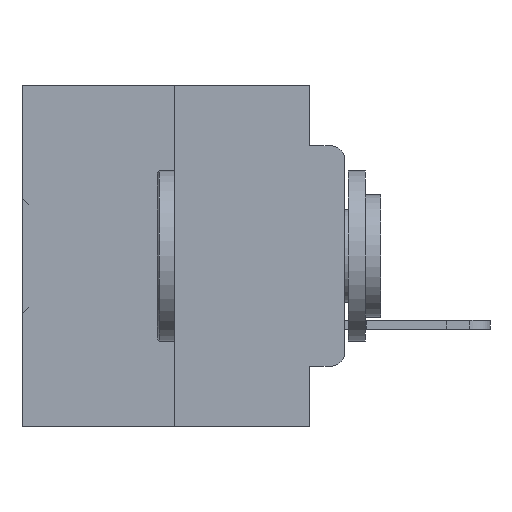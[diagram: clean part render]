
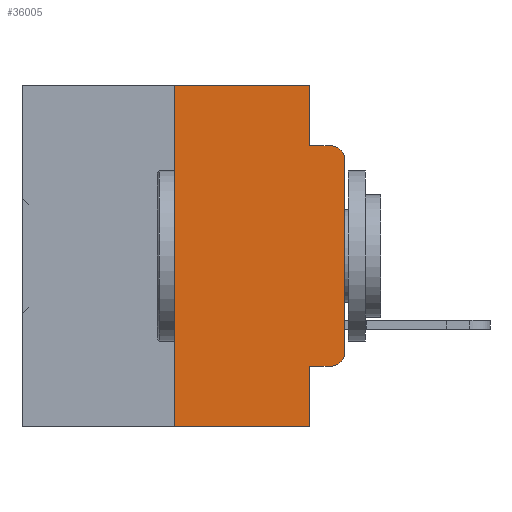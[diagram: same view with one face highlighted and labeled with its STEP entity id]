
A CAD part, left-side view. The second image highlights one B-rep face of the part: STEP entity #36005.
In plain terms, the highlighted planar face has unit normal (-1, 0, 0).
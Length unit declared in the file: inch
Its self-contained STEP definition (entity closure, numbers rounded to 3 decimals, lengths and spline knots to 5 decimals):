
#102 = CIRCLE ( 'NONE', #12698, 0.02 ) ;
#110 = ORIENTED_EDGE ( 'NONE', *, *, #9938, .F. ) ;
#483 = VERTEX_POINT ( 'NONE', #12439 ) ;
#1643 = CARTESIAN_POINT ( 'NONE',  ( 0., 0.051, -0.0885 ) ) ;
#1900 = EDGE_CURVE ( 'NONE', #7193, #11202, #33303, .T. ) ;
#2024 = VECTOR ( 'NONE', #26640, 39.37008 ) ;
#2272 = LINE ( 'NONE', #12925, #31872 ) ;
#2304 = DIRECTION ( 'NONE',  ( 0., -1., 0. ) ) ;
#2772 = DIRECTION ( 'NONE',  ( 0., 0., -1. ) ) ;
#2823 = DIRECTION ( 'NONE',  ( -1., 0., 0. ) ) ;
#2857 = CARTESIAN_POINT ( 'NONE',  ( 0., 0.02, -0.3915 ) ) ;
#3231 = ORIENTED_EDGE ( 'NONE', *, *, #31401, .F. ) ;
#4034 = VERTEX_POINT ( 'NONE', #29962 ) ;
#5088 = CARTESIAN_POINT ( 'NONE',  ( 0., 0., -0.1085 ) ) ;
#5099 = EDGE_CURVE ( 'NONE', #483, #9306, #15165, .T. ) ;
#5623 = EDGE_CURVE ( 'NONE', #483, #21147, #27344, .T. ) ;
#5868 = CARTESIAN_POINT ( 'NONE',  ( 0., 0.473, -0.5 ) ) ;
#7189 = VECTOR ( 'NONE', #19944, 39.37008 ) ;
#7193 = VERTEX_POINT ( 'NONE', #29321 ) ;
#8287 = CARTESIAN_POINT ( 'NONE',  ( 0., 0.02, -0.4115 ) ) ;
#8640 = ORIENTED_EDGE ( 'NONE', *, *, #18039, .F. ) ;
#8737 = VECTOR ( 'NONE', #29853, 39.37008 ) ;
#9306 = VERTEX_POINT ( 'NONE', #8287 ) ;
#9756 = VERTEX_POINT ( 'NONE', #20603 ) ;
#9910 = CARTESIAN_POINT ( 'NONE',  ( 0., 0.473, 0. ) ) ;
#9938 = EDGE_CURVE ( 'NONE', #24594, #34810, #24000, .T. ) ;
#10951 = LINE ( 'NONE', #5868, #25137 ) ;
#11075 = VECTOR ( 'NONE', #14418, 39.37008 ) ;
#11202 = VERTEX_POINT ( 'NONE', #5088 ) ;
#11872 = ORIENTED_EDGE ( 'NONE', *, *, #33392, .F. ) ;
#12439 = CARTESIAN_POINT ( 'NONE',  ( 0., 0.051, -0.4115 ) ) ;
#12698 = AXIS2_PLACEMENT_3D ( 'NONE', #14767, #14762, #14731 ) ;
#12925 = CARTESIAN_POINT ( 'NONE',  ( 0., 0.051, 0. ) ) ;
#13054 = ORIENTED_EDGE ( 'NONE', *, *, #1900, .T. ) ;
#14418 = DIRECTION ( 'NONE',  ( 0., 0., 1. ) ) ;
#14421 = CARTESIAN_POINT ( 'NONE',  ( 0., 0.473, 0. ) ) ;
#14731 = DIRECTION ( 'NONE',  ( 0., 0., -1. ) ) ;
#14754 = DIRECTION ( 'NONE',  ( 0., -1., 0. ) ) ;
#14762 = DIRECTION ( 'NONE',  ( -1., 0., 0. ) ) ;
#14767 = CARTESIAN_POINT ( 'NONE',  ( 0., 0.02, -0.1085 ) ) ;
#15165 = LINE ( 'NONE', #20800, #7189 ) ;
#15496 = ORIENTED_EDGE ( 'NONE', *, *, #29652, .T. ) ;
#15991 = VERTEX_POINT ( 'NONE', #18232 ) ;
#16478 = ORIENTED_EDGE ( 'NONE', *, *, #5623, .F. ) ;
#16813 = EDGE_CURVE ( 'NONE', #9306, #7193, #36131, .T. ) ;
#17270 = DIRECTION ( 'NONE',  ( 0., 0., -1. ) ) ;
#18039 = EDGE_CURVE ( 'NONE', #4034, #15991, #30935, .T. ) ;
#18076 = ORIENTED_EDGE ( 'NONE', *, *, #19427, .T. ) ;
#18232 = CARTESIAN_POINT ( 'NONE',  ( 0., 0.051, 0. ) ) ;
#19427 = EDGE_CURVE ( 'NONE', #11202, #34810, #102, .T. ) ;
#19944 = DIRECTION ( 'NONE',  ( 0., -1., 0. ) ) ;
#20603 = CARTESIAN_POINT ( 'NONE',  ( 0., 0.25, -0.5 ) ) ;
#20800 = CARTESIAN_POINT ( 'NONE',  ( 0., 0.051, -0.4115 ) ) ;
#21147 = VERTEX_POINT ( 'NONE', #35318 ) ;
#22093 = ORIENTED_EDGE ( 'NONE', *, *, #5099, .T. ) ;
#23634 = VECTOR ( 'NONE', #2304, 39.37008 ) ;
#24000 = LINE ( 'NONE', #31769, #8737 ) ;
#24594 = VERTEX_POINT ( 'NONE', #1643 ) ;
#24811 = CARTESIAN_POINT ( 'NONE',  ( 0., 0.02, -0.0885 ) ) ;
#24932 = ORIENTED_EDGE ( 'NONE', *, *, #16813, .T. ) ;
#25137 = VECTOR ( 'NONE', #14754, 39.37008 ) ;
#26344 = AXIS2_PLACEMENT_3D ( 'NONE', #14421, #33726, #17270 ) ;
#26542 = EDGE_LOOP ( 'NONE', ( #13054, #18076, #110, #3231, #8640, #11872, #15496, #16478, #22093, #24932 ) ) ;
#26640 = DIRECTION ( 'NONE',  ( 0., 0., 1. ) ) ;
#26730 = CARTESIAN_POINT ( 'NONE',  ( 0., 0., 0. ) ) ;
#27344 = LINE ( 'NONE', #28347, #34511 ) ;
#28242 = PLANE ( 'NONE',  #26344 ) ;
#28347 = CARTESIAN_POINT ( 'NONE',  ( 0., 0.051, 0. ) ) ;
#29321 = CARTESIAN_POINT ( 'NONE',  ( 0., 0., -0.3915 ) ) ;
#29652 = EDGE_CURVE ( 'NONE', #9756, #21147, #10951, .T. ) ;
#29853 = DIRECTION ( 'NONE',  ( 0., -1., 0. ) ) ;
#29962 = CARTESIAN_POINT ( 'NONE',  ( 0., 0.25, 0. ) ) ;
#30935 = LINE ( 'NONE', #9910, #23634 ) ;
#31056 = DIRECTION ( 'NONE',  ( 0., 0., -1. ) ) ;
#31060 = CARTESIAN_POINT ( 'NONE',  ( 0., 0.25, 0. ) ) ;
#31401 = EDGE_CURVE ( 'NONE', #15991, #24594, #2272, .T. ) ;
#31769 = CARTESIAN_POINT ( 'NONE',  ( 0., 0.051, -0.0885 ) ) ;
#31872 = VECTOR ( 'NONE', #32433, 39.37008 ) ;
#32433 = DIRECTION ( 'NONE',  ( 0., 0., -1. ) ) ;
#33155 = AXIS2_PLACEMENT_3D ( 'NONE', #2857, #2823, #2772 ) ;
#33227 = FACE_OUTER_BOUND ( 'NONE', #26542, .T. ) ;
#33303 = LINE ( 'NONE', #26730, #2024 ) ;
#33392 = EDGE_CURVE ( 'NONE', #9756, #4034, #34176, .T. ) ;
#33726 = DIRECTION ( 'NONE',  ( 1., 0., 0. ) ) ;
#34176 = LINE ( 'NONE', #31060, #11075 ) ;
#34511 = VECTOR ( 'NONE', #31056, 39.37008 ) ;
#34810 = VERTEX_POINT ( 'NONE', #24811 ) ;
#35318 = CARTESIAN_POINT ( 'NONE',  ( 0., 0.051, -0.5 ) ) ;
#36005 = ADVANCED_FACE ( 'NONE', ( #33227 ), #28242, .F. ) ;
#36131 = CIRCLE ( 'NONE', #33155, 0.02 ) ;
